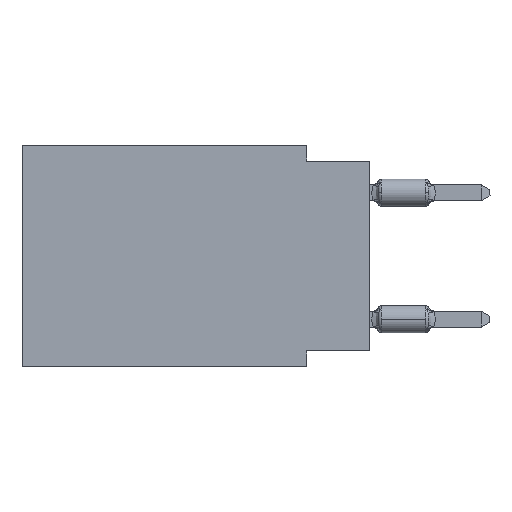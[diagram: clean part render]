
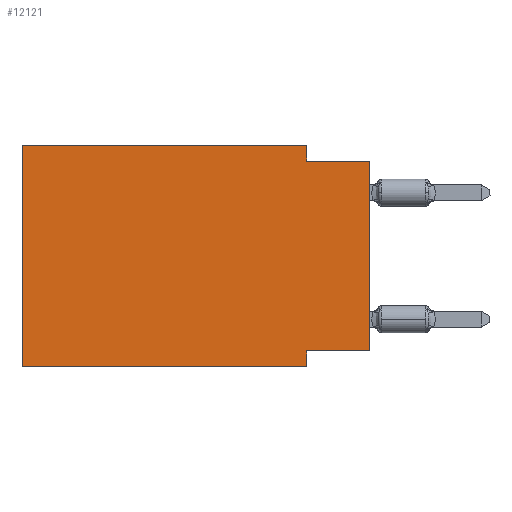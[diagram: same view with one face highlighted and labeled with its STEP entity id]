
A CAD part, left-side view. The second image highlights one B-rep face of the part: STEP entity #12121.
In plain terms, the highlighted planar face has unit normal (-1, 0, 0).
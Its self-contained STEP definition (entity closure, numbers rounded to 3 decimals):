
#160 = ORIENTED_EDGE ( 'NONE', *, *, #9429, .F. ) ;
#527 = VERTEX_POINT ( 'NONE', #10909 ) ;
#558 = VECTOR ( 'NONE', #11921, 1000. ) ;
#1050 = CARTESIAN_POINT ( 'NONE',  ( 0., 2.54, 0. ) ) ;
#1291 = DIRECTION ( 'NONE',  ( 0., 0., -1. ) ) ;
#1391 = CARTESIAN_POINT ( 'NONE',  ( 0., 13.97, -8.89 ) ) ;
#1748 = VECTOR ( 'NONE', #15023, 1000. ) ;
#1932 = VECTOR ( 'NONE', #14276, 1000. ) ;
#2155 = VERTEX_POINT ( 'NONE', #14695 ) ;
#2263 = DIRECTION ( 'NONE',  ( 0., -1., 0. ) ) ;
#2479 = LINE ( 'NONE', #5316, #6930 ) ;
#2697 = EDGE_CURVE ( 'NONE', #18106, #2155, #16589, .T. ) ;
#2818 = EDGE_CURVE ( 'NONE', #527, #7838, #10230, .T. ) ;
#2851 = ORIENTED_EDGE ( 'NONE', *, *, #17882, .F. ) ;
#3124 = VECTOR ( 'NONE', #11872, 1000. ) ;
#3856 = DIRECTION ( 'NONE',  ( 0., 0., 1. ) ) ;
#3967 = CARTESIAN_POINT ( 'NONE',  ( 0., 0., -8.255 ) ) ;
#4736 = CARTESIAN_POINT ( 'NONE',  ( 0., 2.54, -8.89 ) ) ;
#5316 = CARTESIAN_POINT ( 'NONE',  ( 0., 0., -8.255 ) ) ;
#5369 = VECTOR ( 'NONE', #3856, 1000. ) ;
#5502 = LINE ( 'NONE', #11166, #5369 ) ;
#5658 = ORIENTED_EDGE ( 'NONE', *, *, #2818, .F. ) ;
#6559 = VECTOR ( 'NONE', #2263, 1000. ) ;
#6880 = DIRECTION ( 'NONE',  ( 1., 0., 0. ) ) ;
#6930 = VECTOR ( 'NONE', #12185, 1000. ) ;
#7322 = VERTEX_POINT ( 'NONE', #3967 ) ;
#7386 = ORIENTED_EDGE ( 'NONE', *, *, #8899, .F. ) ;
#7537 = CARTESIAN_POINT ( 'NONE',  ( 0., 2.54, 0. ) ) ;
#7661 = EDGE_CURVE ( 'NONE', #7322, #10857, #2479, .T. ) ;
#7838 = VERTEX_POINT ( 'NONE', #17211 ) ;
#8242 = FACE_OUTER_BOUND ( 'NONE', #13600, .T. ) ;
#8745 = AXIS2_PLACEMENT_3D ( 'NONE', #11334, #6880, #1291 ) ;
#8899 = EDGE_CURVE ( 'NONE', #18106, #12344, #5502, .T. ) ;
#9082 = LINE ( 'NONE', #7537, #558 ) ;
#9429 = EDGE_CURVE ( 'NONE', #12344, #12648, #13434, .T. ) ;
#9473 = ORIENTED_EDGE ( 'NONE', *, *, #7661, .F. ) ;
#9494 = ORIENTED_EDGE ( 'NONE', *, *, #11035, .F. ) ;
#10230 = LINE ( 'NONE', #16002, #3124 ) ;
#10857 = VERTEX_POINT ( 'NONE', #18024 ) ;
#10909 = CARTESIAN_POINT ( 'NONE',  ( 0., 2.54, -0.635 ) ) ;
#11035 = EDGE_CURVE ( 'NONE', #10857, #2155, #15896, .T. ) ;
#11166 = CARTESIAN_POINT ( 'NONE',  ( 0., 13.97, 0. ) ) ;
#11334 = CARTESIAN_POINT ( 'NONE',  ( 0., 13.97, 0. ) ) ;
#11872 = DIRECTION ( 'NONE',  ( 0., -1., 0. ) ) ;
#11921 = DIRECTION ( 'NONE',  ( 0., 0., -1. ) ) ;
#11980 = EDGE_CURVE ( 'NONE', #7322, #7838, #16487, .T. ) ;
#12121 = ADVANCED_FACE ( 'NONE', ( #8242 ), #14173, .F. ) ;
#12139 = CARTESIAN_POINT ( 'NONE',  ( 0., 13.97, 0. ) ) ;
#12185 = DIRECTION ( 'NONE',  ( 0., 1., 0. ) ) ;
#12344 = VERTEX_POINT ( 'NONE', #12139 ) ;
#12648 = VERTEX_POINT ( 'NONE', #1050 ) ;
#13163 = CARTESIAN_POINT ( 'NONE',  ( 0., 13.97, 0. ) ) ;
#13434 = LINE ( 'NONE', #13163, #6559 ) ;
#13600 = EDGE_LOOP ( 'NONE', ( #16610, #5658, #2851, #160, #7386, #13766, #9494, #9473 ) ) ;
#13664 = CARTESIAN_POINT ( 'NONE',  ( 0., 13.97, -8.89 ) ) ;
#13766 = ORIENTED_EDGE ( 'NONE', *, *, #2697, .T. ) ;
#14173 = PLANE ( 'NONE',  #8745 ) ;
#14276 = DIRECTION ( 'NONE',  ( 0., -1., 0. ) ) ;
#14590 = VECTOR ( 'NONE', #14895, 1000. ) ;
#14695 = CARTESIAN_POINT ( 'NONE',  ( 0., 2.54, -8.89 ) ) ;
#14895 = DIRECTION ( 'NONE',  ( 0., 0., -1. ) ) ;
#15023 = DIRECTION ( 'NONE',  ( 0., 0., 1. ) ) ;
#15896 = LINE ( 'NONE', #4736, #14590 ) ;
#16002 = CARTESIAN_POINT ( 'NONE',  ( 0., 0., -0.635 ) ) ;
#16487 = LINE ( 'NONE', #17952, #1748 ) ;
#16589 = LINE ( 'NONE', #13664, #1932 ) ;
#16610 = ORIENTED_EDGE ( 'NONE', *, *, #11980, .T. ) ;
#17211 = CARTESIAN_POINT ( 'NONE',  ( 0., 0., -0.635 ) ) ;
#17882 = EDGE_CURVE ( 'NONE', #12648, #527, #9082, .T. ) ;
#17952 = CARTESIAN_POINT ( 'NONE',  ( 0., 0., 0. ) ) ;
#18024 = CARTESIAN_POINT ( 'NONE',  ( 0., 2.54, -8.255 ) ) ;
#18106 = VERTEX_POINT ( 'NONE', #1391 ) ;
